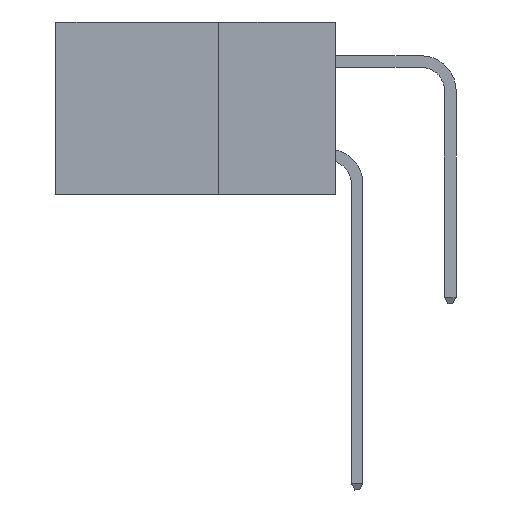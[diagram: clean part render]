
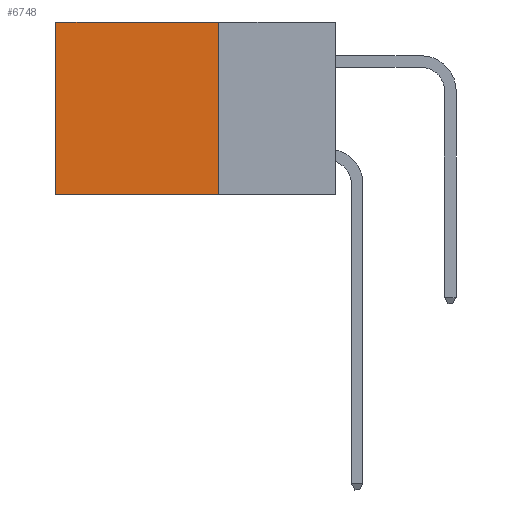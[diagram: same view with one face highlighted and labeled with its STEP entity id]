
A CAD part, left-side view. The second image highlights one B-rep face of the part: STEP entity #6748.
In plain terms, the highlighted planar face has unit normal (-1, 0, 0).
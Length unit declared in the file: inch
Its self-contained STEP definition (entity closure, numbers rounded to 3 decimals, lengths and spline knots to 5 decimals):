
#40 = CARTESIAN_POINT ( 'NONE',  ( 0.2875, 0.25, 0. ) ) ;
#233 = VERTEX_POINT ( 'NONE', #19298 ) ;
#1175 = EDGE_CURVE ( 'NONE', #233, #21010, #33169, .T. ) ;
#1286 = LINE ( 'NONE', #33877, #31894 ) ;
#2673 = CARTESIAN_POINT ( 'NONE',  ( 0.2875, 0.6, 0. ) ) ;
#3955 = DIRECTION ( 'NONE',  ( 0., 0., -1. ) ) ;
#4981 = CARTESIAN_POINT ( 'NONE',  ( 0.2875, 0.6, -0.37 ) ) ;
#5426 = CARTESIAN_POINT ( 'NONE',  ( 0.2875, 0.25, -0.37 ) ) ;
#5697 = DIRECTION ( 'NONE',  ( 0., 1., 0. ) ) ;
#6061 = ORIENTED_EDGE ( 'NONE', *, *, #1175, .T. ) ;
#6748 = ADVANCED_FACE ( 'NONE', ( #22732 ), #16227, .F. ) ;
#7561 = ORIENTED_EDGE ( 'NONE', *, *, #20384, .F. ) ;
#7970 = DIRECTION ( 'NONE',  ( 1., 0., 0. ) ) ;
#9193 = DIRECTION ( 'NONE',  ( 0., 1., 0. ) ) ;
#12603 = EDGE_CURVE ( 'NONE', #18116, #233, #18339, .T. ) ;
#14794 = VERTEX_POINT ( 'NONE', #34416 ) ;
#16227 = PLANE ( 'NONE',  #33915 ) ;
#16427 = VECTOR ( 'NONE', #20445, 39.37008 ) ;
#18116 = VERTEX_POINT ( 'NONE', #33178 ) ;
#18339 = LINE ( 'NONE', #40, #23446 ) ;
#19298 = CARTESIAN_POINT ( 'NONE',  ( 0.2875, 0.6, 0. ) ) ;
#20384 = EDGE_CURVE ( 'NONE', #14794, #21010, #32649, .T. ) ;
#20445 = DIRECTION ( 'NONE',  ( 0., 0., -1. ) ) ;
#20600 = VECTOR ( 'NONE', #5697, 39.37008 ) ;
#21010 = VERTEX_POINT ( 'NONE', #4981 ) ;
#22732 = FACE_OUTER_BOUND ( 'NONE', #29042, .T. ) ;
#23446 = VECTOR ( 'NONE', #9193, 39.37008 ) ;
#24726 = ORIENTED_EDGE ( 'NONE', *, *, #12603, .T. ) ;
#25109 = ORIENTED_EDGE ( 'NONE', *, *, #27217, .F. ) ;
#27217 = EDGE_CURVE ( 'NONE', #18116, #14794, #1286, .T. ) ;
#29042 = EDGE_LOOP ( 'NONE', ( #6061, #7561, #25109, #24726 ) ) ;
#29053 = CARTESIAN_POINT ( 'NONE',  ( 0.2875, 0.25, 0. ) ) ;
#31894 = VECTOR ( 'NONE', #3955, 39.37008 ) ;
#32649 = LINE ( 'NONE', #5426, #20600 ) ;
#33169 = LINE ( 'NONE', #2673, #16427 ) ;
#33178 = CARTESIAN_POINT ( 'NONE',  ( 0.2875, 0.25, 0. ) ) ;
#33877 = CARTESIAN_POINT ( 'NONE',  ( 0.2875, 0.25, 0. ) ) ;
#33915 = AXIS2_PLACEMENT_3D ( 'NONE', #29053, #7970, #38226 ) ;
#34416 = CARTESIAN_POINT ( 'NONE',  ( 0.2875, 0.25, -0.37 ) ) ;
#38226 = DIRECTION ( 'NONE',  ( 0., 0., -1. ) ) ;
